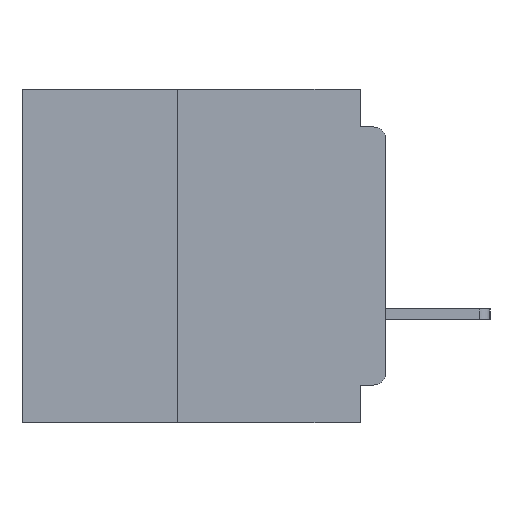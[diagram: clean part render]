
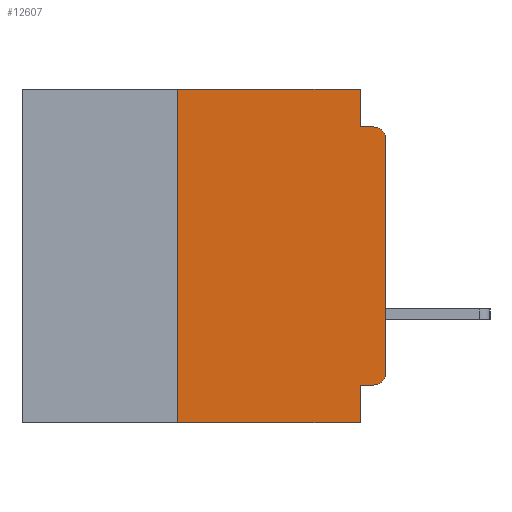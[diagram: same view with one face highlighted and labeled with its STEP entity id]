
A CAD part, left-side view. The second image highlights one B-rep face of the part: STEP entity #12607.
In plain terms, the highlighted planar face has unit normal (-1, 0, 0).
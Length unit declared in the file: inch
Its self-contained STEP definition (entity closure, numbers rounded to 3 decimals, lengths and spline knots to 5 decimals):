
#717 = ORIENTED_EDGE ( 'NONE', *, *, #50969, .F. ) ;
#987 = CARTESIAN_POINT ( 'NONE',  ( 0., 0.437, -0.4 ) ) ;
#998 = DIRECTION ( 'NONE',  ( 0., 0., 1. ) ) ;
#1314 = CARTESIAN_POINT ( 'NONE',  ( 0., 0.015, -0.355 ) ) ;
#1536 = ORIENTED_EDGE ( 'NONE', *, *, #50481, .F. ) ;
#1626 = CARTESIAN_POINT ( 'NONE',  ( 0., 0., -0.355 ) ) ;
#2678 = EDGE_CURVE ( 'NONE', #23734, #21491, #8705, .T. ) ;
#3351 = DIRECTION ( 'NONE',  ( 1., 0., 0. ) ) ;
#3840 = CARTESIAN_POINT ( 'NONE',  ( 0., 0.031, -0.045 ) ) ;
#7069 = DIRECTION ( 'NONE',  ( 0., -1., 0. ) ) ;
#7167 = VECTOR ( 'NONE', #44230, 39.37008 ) ;
#7603 = CARTESIAN_POINT ( 'NONE',  ( 0., 0.031, 0. ) ) ;
#8319 = VERTEX_POINT ( 'NONE', #3840 ) ;
#8705 = LINE ( 'NONE', #45117, #7167 ) ;
#10044 = CARTESIAN_POINT ( 'NONE',  ( 0., 0., -0.045 ) ) ;
#10173 = CARTESIAN_POINT ( 'NONE',  ( 0., 0.015, -0.06 ) ) ;
#11003 = VECTOR ( 'NONE', #63977, 39.37008 ) ;
#11031 = ORIENTED_EDGE ( 'NONE', *, *, #56223, .F. ) ;
#12573 = LINE ( 'NONE', #19123, #11003 ) ;
#12607 = ADVANCED_FACE ( 'NONE', ( #45921 ), #28070, .F. ) ;
#13256 = VERTEX_POINT ( 'NONE', #52955 ) ;
#14937 = LINE ( 'NONE', #41610, #41200 ) ;
#15022 = DIRECTION ( 'NONE',  ( 0., -1., 0. ) ) ;
#15110 = CARTESIAN_POINT ( 'NONE',  ( 0., 0., -0.34 ) ) ;
#15150 = DIRECTION ( 'NONE',  ( 0., 0., -1. ) ) ;
#16697 = LINE ( 'NONE', #50508, #28366 ) ;
#16822 = VERTEX_POINT ( 'NONE', #35545 ) ;
#18087 = CARTESIAN_POINT ( 'NONE',  ( 0., 0.015, -0.34 ) ) ;
#18788 = VECTOR ( 'NONE', #41217, 39.37008 ) ;
#19123 = CARTESIAN_POINT ( 'NONE',  ( 0., 0., 0. ) ) ;
#20092 = ORIENTED_EDGE ( 'NONE', *, *, #24623, .T. ) ;
#20517 = EDGE_CURVE ( 'NONE', #8319, #13256, #45540, .T. ) ;
#21491 = VERTEX_POINT ( 'NONE', #59782 ) ;
#23010 = ORIENTED_EDGE ( 'NONE', *, *, #2678, .F. ) ;
#23093 = DIRECTION ( 'NONE',  ( 0., 0., -1. ) ) ;
#23734 = VERTEX_POINT ( 'NONE', #61872 ) ;
#23823 = CARTESIAN_POINT ( 'NONE',  ( 0., 0.25, -0.4 ) ) ;
#23926 = AXIS2_PLACEMENT_3D ( 'NONE', #10173, #44712, #15150 ) ;
#24623 = EDGE_CURVE ( 'NONE', #16822, #13256, #59383, .T. ) ;
#24666 = AXIS2_PLACEMENT_3D ( 'NONE', #18087, #52611, #23093 ) ;
#25825 = VERTEX_POINT ( 'NONE', #39608 ) ;
#27513 = ORIENTED_EDGE ( 'NONE', *, *, #61305, .T. ) ;
#27623 = VERTEX_POINT ( 'NONE', #15110 ) ;
#28070 = PLANE ( 'NONE',  #53247 ) ;
#28366 = VECTOR ( 'NONE', #998, 39.37008 ) ;
#30932 = VECTOR ( 'NONE', #15022, 39.37008 ) ;
#31678 = VECTOR ( 'NONE', #45505, 39.37008 ) ;
#31947 = LINE ( 'NONE', #1626, #18788 ) ;
#32899 = CIRCLE ( 'NONE', #24666, 0.015 ) ;
#33702 = CARTESIAN_POINT ( 'NONE',  ( 0., 0.031, 0. ) ) ;
#33796 = VERTEX_POINT ( 'NONE', #1314 ) ;
#35545 = CARTESIAN_POINT ( 'NONE',  ( 0., 0., -0.06 ) ) ;
#36361 = EDGE_LOOP ( 'NONE', ( #27513, #20092, #60068, #1536, #11031, #53176, #43152, #23010, #717, #63291 ) ) ;
#37980 = DIRECTION ( 'NONE',  ( 0., 0., -1. ) ) ;
#39608 = CARTESIAN_POINT ( 'NONE',  ( 0., 0.25, 0. ) ) ;
#41200 = VECTOR ( 'NONE', #7069, 39.37008 ) ;
#41217 = DIRECTION ( 'NONE',  ( 0., 1., 0. ) ) ;
#41610 = CARTESIAN_POINT ( 'NONE',  ( 0., 0.437, 0. ) ) ;
#42816 = LINE ( 'NONE', #7603, #62862 ) ;
#43152 = ORIENTED_EDGE ( 'NONE', *, *, #46779, .T. ) ;
#44230 = DIRECTION ( 'NONE',  ( 0., 0., -1. ) ) ;
#44712 = DIRECTION ( 'NONE',  ( -1., 0., 0. ) ) ;
#44767 = LINE ( 'NONE', #987, #31678 ) ;
#45117 = CARTESIAN_POINT ( 'NONE',  ( 0., 0.031, -0.4 ) ) ;
#45505 = DIRECTION ( 'NONE',  ( 0., -1., 0. ) ) ;
#45540 = LINE ( 'NONE', #10044, #30932 ) ;
#45921 = FACE_OUTER_BOUND ( 'NONE', #36361, .T. ) ;
#46779 = EDGE_CURVE ( 'NONE', #63583, #21491, #44767, .T. ) ;
#47081 = DIRECTION ( 'NONE',  ( 0., 0., -1. ) ) ;
#48590 = EDGE_CURVE ( 'NONE', #63583, #25825, #16697, .T. ) ;
#50481 = EDGE_CURVE ( 'NONE', #53257, #8319, #42816, .T. ) ;
#50508 = CARTESIAN_POINT ( 'NONE',  ( 0., 0.25, -0.4 ) ) ;
#50969 = EDGE_CURVE ( 'NONE', #33796, #23734, #31947, .T. ) ;
#52611 = DIRECTION ( 'NONE',  ( -1., 0., 0. ) ) ;
#52955 = CARTESIAN_POINT ( 'NONE',  ( 0., 0.015, -0.045 ) ) ;
#53176 = ORIENTED_EDGE ( 'NONE', *, *, #48590, .F. ) ;
#53247 = AXIS2_PLACEMENT_3D ( 'NONE', #62532, #3351, #37980 ) ;
#53257 = VERTEX_POINT ( 'NONE', #33702 ) ;
#56223 = EDGE_CURVE ( 'NONE', #25825, #53257, #14937, .T. ) ;
#59383 = CIRCLE ( 'NONE', #23926, 0.015 ) ;
#59782 = CARTESIAN_POINT ( 'NONE',  ( 0., 0.031, -0.4 ) ) ;
#60068 = ORIENTED_EDGE ( 'NONE', *, *, #20517, .F. ) ;
#60124 = EDGE_CURVE ( 'NONE', #33796, #27623, #32899, .T. ) ;
#61305 = EDGE_CURVE ( 'NONE', #27623, #16822, #12573, .T. ) ;
#61872 = CARTESIAN_POINT ( 'NONE',  ( 0., 0.031, -0.355 ) ) ;
#62532 = CARTESIAN_POINT ( 'NONE',  ( 0., 0.437, 0. ) ) ;
#62862 = VECTOR ( 'NONE', #47081, 39.37008 ) ;
#63291 = ORIENTED_EDGE ( 'NONE', *, *, #60124, .T. ) ;
#63583 = VERTEX_POINT ( 'NONE', #23823 ) ;
#63977 = DIRECTION ( 'NONE',  ( 0., 0., 1. ) ) ;
